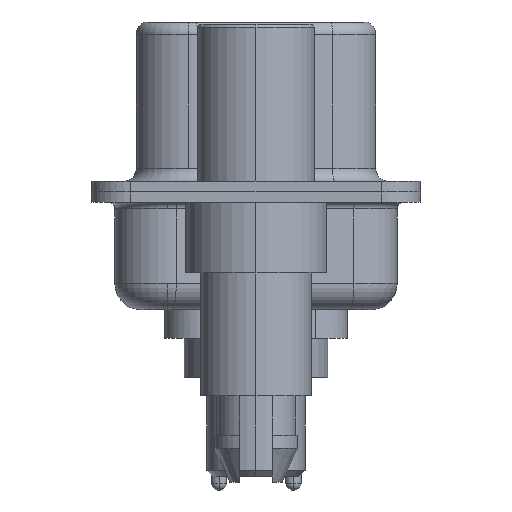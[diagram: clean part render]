
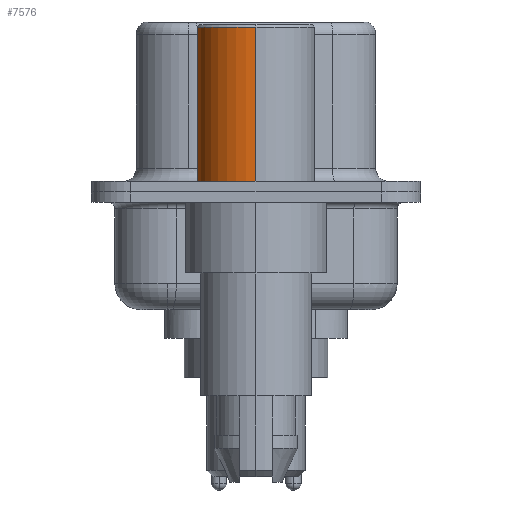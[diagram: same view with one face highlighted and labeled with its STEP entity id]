
A CAD part, left-side view. The second image highlights one B-rep face of the part: STEP entity #7576.
In plain terms, the highlighted cylindrical face has radius 2.25 mm (diameter 4.5 mm), a partial arc.
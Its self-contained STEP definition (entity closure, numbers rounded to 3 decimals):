
#1115 = CYLINDRICAL_SURFACE ( 'NONE', #7380, 2.25 ) ;
#1492 = DIRECTION ( 'NONE',  ( 0., 0., 1. ) ) ;
#1714 = CARTESIAN_POINT ( 'NONE',  ( 0., 0., 6.3 ) ) ;
#2129 = LINE ( 'NONE', #7368, #8591 ) ;
#2145 = CARTESIAN_POINT ( 'NONE',  ( -2.25, 0., 0.4 ) ) ;
#2226 = ORIENTED_EDGE ( 'NONE', *, *, #15657, .F. ) ;
#2445 = CARTESIAN_POINT ( 'NONE',  ( 2.25, 0., 0.4 ) ) ;
#2595 = ORIENTED_EDGE ( 'NONE', *, *, #8430, .T. ) ;
#2927 = DIRECTION ( 'NONE',  ( 1., 0., 0. ) ) ;
#3074 = CARTESIAN_POINT ( 'NONE',  ( 2.25, 0., 6.3 ) ) ;
#4443 = AXIS2_PLACEMENT_3D ( 'NONE', #1714, #10645, #2927 ) ;
#4565 = DIRECTION ( 'NONE',  ( 0., 0., 1. ) ) ;
#4580 = EDGE_CURVE ( 'NONE', #15317, #7547, #2129, .T. ) ;
#5591 = ORIENTED_EDGE ( 'NONE', *, *, #8534, .T. ) ;
#5719 = DIRECTION ( 'NONE',  ( 0., 0., 1. ) ) ;
#7057 = DIRECTION ( 'NONE',  ( 1., 0., 0. ) ) ;
#7368 = CARTESIAN_POINT ( 'NONE',  ( 2.25, 0., 0.581 ) ) ;
#7380 = AXIS2_PLACEMENT_3D ( 'NONE', #15633, #5719, #7057 ) ;
#7547 = VERTEX_POINT ( 'NONE', #3074 ) ;
#7576 = ADVANCED_FACE ( 'NONE', ( #11220 ), #1115, .T. ) ;
#7889 = EDGE_LOOP ( 'NONE', ( #5591, #2595, #2226, #12609 ) ) ;
#8221 = DIRECTION ( 'NONE',  ( 0., 0., 1. ) ) ;
#8430 = EDGE_CURVE ( 'NONE', #13572, #9947, #11190, .T. ) ;
#8534 = EDGE_CURVE ( 'NONE', #15317, #13572, #8863, .T. ) ;
#8591 = VECTOR ( 'NONE', #1492, 1000. ) ;
#8863 = CIRCLE ( 'NONE', #12500, 2.25 ) ;
#9947 = VERTEX_POINT ( 'NONE', #13964 ) ;
#10645 = DIRECTION ( 'NONE',  ( 0., 0., 1. ) ) ;
#11190 = LINE ( 'NONE', #15532, #11558 ) ;
#11220 = FACE_OUTER_BOUND ( 'NONE', #7889, .T. ) ;
#11558 = VECTOR ( 'NONE', #8221, 1000. ) ;
#12223 = CARTESIAN_POINT ( 'NONE',  ( 0., 0., 0.4 ) ) ;
#12500 = AXIS2_PLACEMENT_3D ( 'NONE', #12223, #4565, #13435 ) ;
#12609 = ORIENTED_EDGE ( 'NONE', *, *, #4580, .F. ) ;
#13435 = DIRECTION ( 'NONE',  ( 1., 0., 0. ) ) ;
#13572 = VERTEX_POINT ( 'NONE', #2145 ) ;
#13764 = CIRCLE ( 'NONE', #4443, 2.25 ) ;
#13964 = CARTESIAN_POINT ( 'NONE',  ( -2.25, 0., 6.3 ) ) ;
#15317 = VERTEX_POINT ( 'NONE', #2445 ) ;
#15532 = CARTESIAN_POINT ( 'NONE',  ( -2.25, 0., 0.581 ) ) ;
#15633 = CARTESIAN_POINT ( 'NONE',  ( 0., 0., 0.581 ) ) ;
#15657 = EDGE_CURVE ( 'NONE', #7547, #9947, #13764, .T. ) ;
